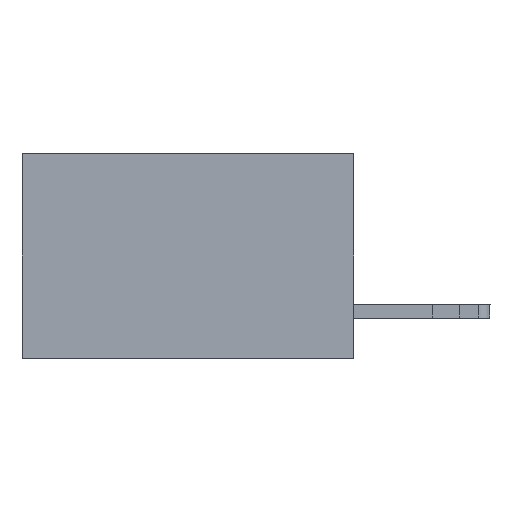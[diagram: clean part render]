
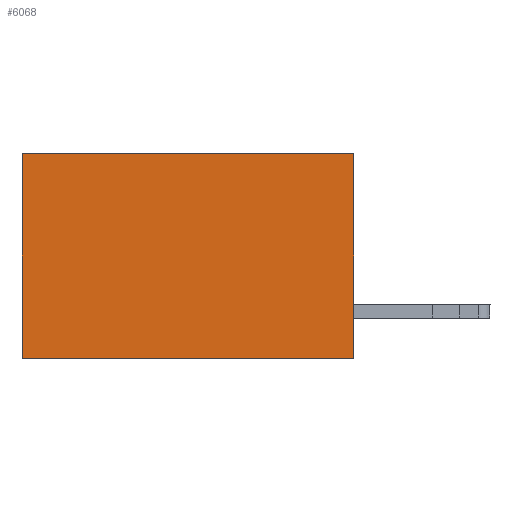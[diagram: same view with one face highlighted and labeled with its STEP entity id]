
A CAD part, left-side view. The second image highlights one B-rep face of the part: STEP entity #6068.
In plain terms, the highlighted planar face has unit normal (-1, 0, 0).
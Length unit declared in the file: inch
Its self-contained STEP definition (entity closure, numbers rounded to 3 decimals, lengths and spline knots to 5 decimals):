
#97 = VERTEX_POINT ( 'NONE', #6701 ) ;
#257 = DIRECTION ( 'NONE',  ( 0., 0., -1. ) ) ;
#336 = DIRECTION ( 'NONE',  ( 1., 0., 0. ) ) ;
#369 = VECTOR ( 'NONE', #5980, 39.37008 ) ;
#537 = CARTESIAN_POINT ( 'NONE',  ( 0.2875, 0., 0. ) ) ;
#1364 = ORIENTED_EDGE ( 'NONE', *, *, #15620, .F. ) ;
#1450 = AXIS2_PLACEMENT_3D ( 'NONE', #17002, #336, #18436 ) ;
#2335 = DIRECTION ( 'NONE',  ( 0., 1., 0. ) ) ;
#5211 = PLANE ( 'NONE',  #1450 ) ;
#5466 = VECTOR ( 'NONE', #9053, 39.37008 ) ;
#5980 = DIRECTION ( 'NONE',  ( 0., 0., -1. ) ) ;
#6068 = ADVANCED_FACE ( 'NONE', ( #20962 ), #5211, .F. ) ;
#6701 = CARTESIAN_POINT ( 'NONE',  ( 0.2875, 0., 0. ) ) ;
#6752 = LINE ( 'NONE', #17257, #5466 ) ;
#7156 = EDGE_CURVE ( 'NONE', #13815, #8511, #17127, .T. ) ;
#8511 = VERTEX_POINT ( 'NONE', #15067 ) ;
#8947 = VECTOR ( 'NONE', #257, 39.37008 ) ;
#8969 = LINE ( 'NONE', #537, #14107 ) ;
#9053 = DIRECTION ( 'NONE',  ( 0., 1., 0. ) ) ;
#12883 = CARTESIAN_POINT ( 'NONE',  ( 0.2875, 0., -0.37 ) ) ;
#12924 = EDGE_CURVE ( 'NONE', #97, #16974, #18455, .T. ) ;
#13086 = EDGE_CURVE ( 'NONE', #97, #13815, #8969, .T. ) ;
#13815 = VERTEX_POINT ( 'NONE', #17482 ) ;
#14107 = VECTOR ( 'NONE', #2335, 39.37008 ) ;
#14897 = ORIENTED_EDGE ( 'NONE', *, *, #7156, .T. ) ;
#15043 = CARTESIAN_POINT ( 'NONE',  ( 0.2875, 0., 0. ) ) ;
#15048 = ORIENTED_EDGE ( 'NONE', *, *, #13086, .T. ) ;
#15067 = CARTESIAN_POINT ( 'NONE',  ( 0.2875, 0.6, -0.37 ) ) ;
#15620 = EDGE_CURVE ( 'NONE', #16974, #8511, #6752, .T. ) ;
#16974 = VERTEX_POINT ( 'NONE', #12883 ) ;
#17002 = CARTESIAN_POINT ( 'NONE',  ( 0.2875, 0., 0. ) ) ;
#17127 = LINE ( 'NONE', #19468, #369 ) ;
#17257 = CARTESIAN_POINT ( 'NONE',  ( 0.2875, 0., -0.37 ) ) ;
#17482 = CARTESIAN_POINT ( 'NONE',  ( 0.2875, 0.6, 0. ) ) ;
#17912 = EDGE_LOOP ( 'NONE', ( #14897, #1364, #20698, #15048 ) ) ;
#18436 = DIRECTION ( 'NONE',  ( 0., 0., -1. ) ) ;
#18455 = LINE ( 'NONE', #15043, #8947 ) ;
#19468 = CARTESIAN_POINT ( 'NONE',  ( 0.2875, 0.6, 0. ) ) ;
#20698 = ORIENTED_EDGE ( 'NONE', *, *, #12924, .F. ) ;
#20962 = FACE_OUTER_BOUND ( 'NONE', #17912, .T. ) ;
